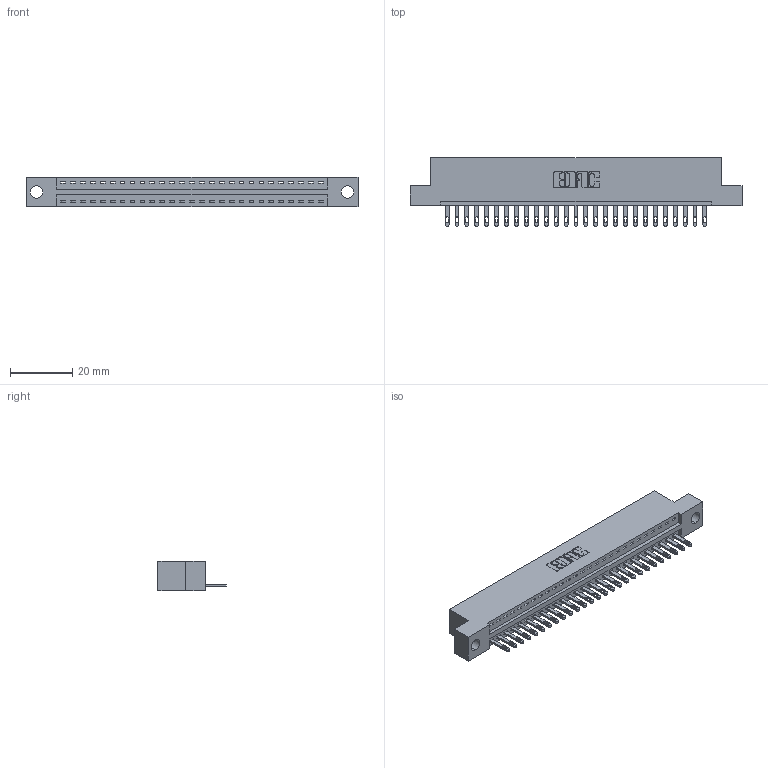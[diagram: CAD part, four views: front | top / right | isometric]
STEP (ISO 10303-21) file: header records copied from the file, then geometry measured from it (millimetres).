
FILE_DESCRIPTION (( 'STEP AP203' ), '1' );
FILE_NAME ('346-027-500-104.STEP', '2022-05-06T03:47:59', ( '' ), ( '' ), 'SwSTEP 2.0', 'SolidWorks 2020', '' );
FILE_SCHEMA (( 'CONFIG_CONTROL_DESIGN' ));
Length unit declared in the file: inch
Products named in the file (3): 346 Part_Flush Mounting Lugs - 0.156 Dia-TH; 345-292-001_345-293-100; 346-027-500-104
Assembly tree (28 placements, depth 2):
  346-027-500-104
    346 Part_Flush Mounting Lugs - 0.156 Dia-TH
    345-292-001_345-293-100  x27
Bounding box: 106.3 x 21.84 x 9.4 mm (x, y, z)
Volume: 9982.6 mm3; surface area: 12215.2 mm2
Topology: 28 solids, 28 shells, 1594 faces, 4901 edges, 3266 vertices
Faces by surface type: plane 1008, cylinder 586
Entity records: 19125 total; most frequent: CARTESIAN_POINT 3291, ORIENTED_EDGE 3250, DIRECTION 2923, EDGE_CURVE 1625, LINE 1381, VECTOR 1381, VERTEX_POINT 1082, AXIS2_PLACEMENT_3D 771
